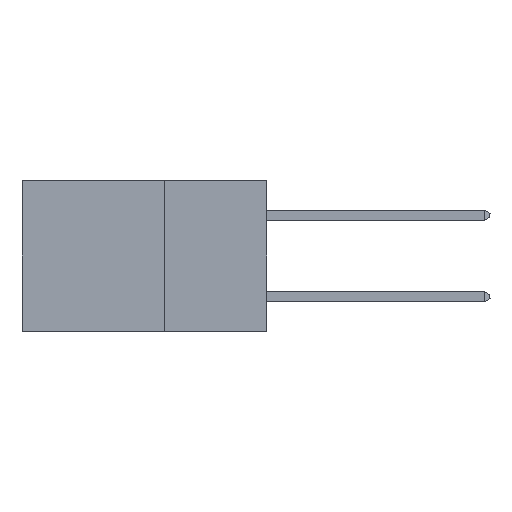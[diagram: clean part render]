
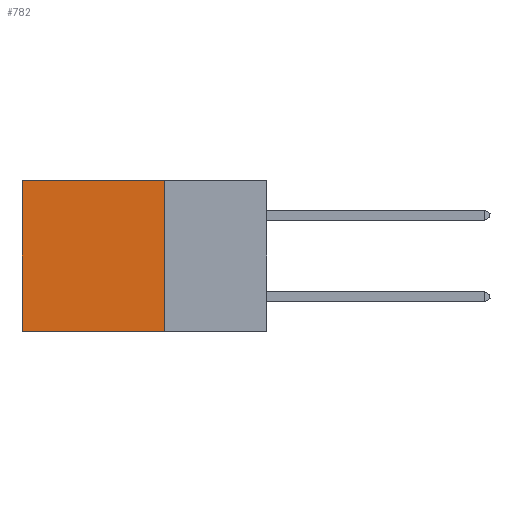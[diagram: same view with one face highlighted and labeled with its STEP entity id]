
A CAD part, left-side view. The second image highlights one B-rep face of the part: STEP entity #782.
In plain terms, the highlighted planar face has unit normal (-1, 0, 0).
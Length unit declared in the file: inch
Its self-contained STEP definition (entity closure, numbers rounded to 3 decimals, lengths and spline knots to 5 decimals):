
#782 = ADVANCED_FACE ( 'NONE', ( #23126 ), #2564, .F. ) ;
#1024 = LINE ( 'NONE', #33492, #19502 ) ;
#2564 = PLANE ( 'NONE',  #10854 ) ;
#3572 = VERTEX_POINT ( 'NONE', #31084 ) ;
#4569 = DIRECTION ( 'NONE',  ( 0., 0., -1. ) ) ;
#4937 = EDGE_CURVE ( 'NONE', #24313, #3572, #16341, .T. ) ;
#5519 = CARTESIAN_POINT ( 'NONE',  ( 0.2875, 0.25, 0. ) ) ;
#7334 = CARTESIAN_POINT ( 'NONE',  ( 0.2875, 0.25, 0. ) ) ;
#7958 = VERTEX_POINT ( 'NONE', #7334 ) ;
#8201 = DIRECTION ( 'NONE',  ( 0., 1., 0. ) ) ;
#8510 = VECTOR ( 'NONE', #15031, 39.37008 ) ;
#9020 = ORIENTED_EDGE ( 'NONE', *, *, #36402, .T. ) ;
#9426 = LINE ( 'NONE', #22133, #12641 ) ;
#10854 = AXIS2_PLACEMENT_3D ( 'NONE', #5519, #23831, #18425 ) ;
#12641 = VECTOR ( 'NONE', #4569, 39.37008 ) ;
#13574 = DIRECTION ( 'NONE',  ( 0., 0., -1. ) ) ;
#13837 = EDGE_LOOP ( 'NONE', ( #9020, #32682, #24581, #29938 ) ) ;
#15031 = DIRECTION ( 'NONE',  ( 0., 1., 0. ) ) ;
#15937 = EDGE_CURVE ( 'NONE', #7958, #31596, #1024, .T. ) ;
#16341 = LINE ( 'NONE', #26790, #8510 ) ;
#17734 = VECTOR ( 'NONE', #13574, 39.37008 ) ;
#18425 = DIRECTION ( 'NONE',  ( 0., 0., -1. ) ) ;
#19502 = VECTOR ( 'NONE', #8201, 39.37008 ) ;
#22133 = CARTESIAN_POINT ( 'NONE',  ( 0.2875, 0.25, 0. ) ) ;
#22789 = CARTESIAN_POINT ( 'NONE',  ( 0.2875, 0.6, 0. ) ) ;
#23126 = FACE_OUTER_BOUND ( 'NONE', #13837, .T. ) ;
#23831 = DIRECTION ( 'NONE',  ( 1., 0., 0. ) ) ;
#24313 = VERTEX_POINT ( 'NONE', #24724 ) ;
#24581 = ORIENTED_EDGE ( 'NONE', *, *, #36221, .F. ) ;
#24724 = CARTESIAN_POINT ( 'NONE',  ( 0.2875, 0.25, -0.37 ) ) ;
#26790 = CARTESIAN_POINT ( 'NONE',  ( 0.2875, 0.25, -0.37 ) ) ;
#29938 = ORIENTED_EDGE ( 'NONE', *, *, #15937, .T. ) ;
#31084 = CARTESIAN_POINT ( 'NONE',  ( 0.2875, 0.6, -0.37 ) ) ;
#31596 = VERTEX_POINT ( 'NONE', #34266 ) ;
#32682 = ORIENTED_EDGE ( 'NONE', *, *, #4937, .F. ) ;
#33492 = CARTESIAN_POINT ( 'NONE',  ( 0.2875, 0.25, 0. ) ) ;
#34266 = CARTESIAN_POINT ( 'NONE',  ( 0.2875, 0.6, 0. ) ) ;
#36221 = EDGE_CURVE ( 'NONE', #7958, #24313, #9426, .T. ) ;
#36402 = EDGE_CURVE ( 'NONE', #31596, #3572, #38057, .T. ) ;
#38057 = LINE ( 'NONE', #22789, #17734 ) ;
